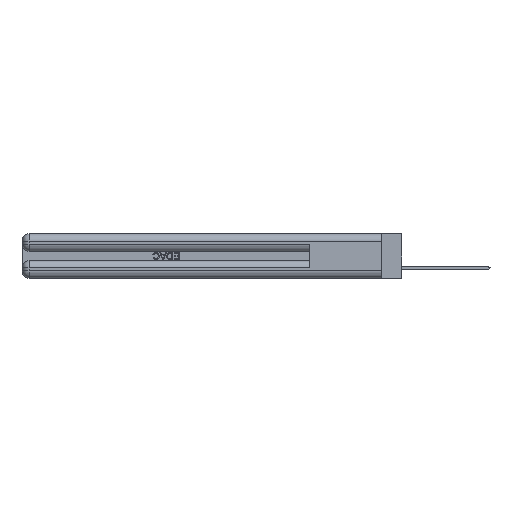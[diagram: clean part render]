
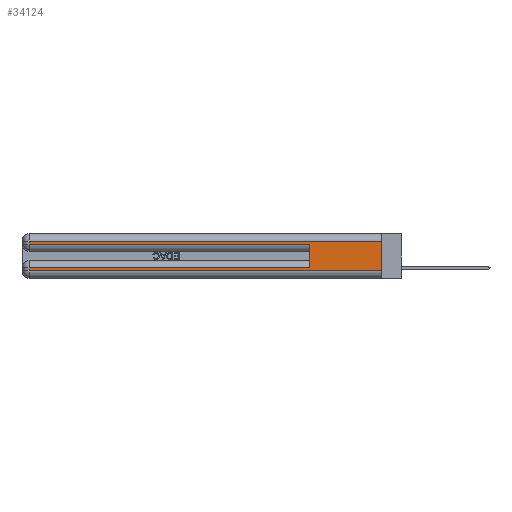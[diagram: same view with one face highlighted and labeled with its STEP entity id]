
A CAD part, left-side view. The second image highlights one B-rep face of the part: STEP entity #34124.
In plain terms, the highlighted planar face has unit normal (-1, 0, 0).
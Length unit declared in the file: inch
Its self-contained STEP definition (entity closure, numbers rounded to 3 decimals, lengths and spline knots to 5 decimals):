
#1378 = ORIENTED_EDGE ( 'NONE', *, *, #38649, .T. ) ;
#1786 = PLANE ( 'NONE',  #33733 ) ;
#1839 = CARTESIAN_POINT ( 'NONE',  ( 0., 2.94, 0.06 ) ) ;
#2216 = CARTESIAN_POINT ( 'NONE',  ( 0., 2.94, 0.085 ) ) ;
#2535 = ORIENTED_EDGE ( 'NONE', *, *, #29352, .T. ) ;
#3140 = CARTESIAN_POINT ( 'NONE',  ( 0., 0., 0.31 ) ) ;
#3660 = EDGE_CURVE ( 'NONE', #37963, #29815, #36804, .T. ) ;
#3830 = LINE ( 'NONE', #30878, #46070 ) ;
#4419 = EDGE_CURVE ( 'NONE', #34968, #53987, #10889, .T. ) ;
#8292 = VECTOR ( 'NONE', #16540, 39.37008 ) ;
#9470 = LINE ( 'NONE', #28922, #42592 ) ;
#9573 = CARTESIAN_POINT ( 'NONE',  ( 0., 0., 0.37 ) ) ;
#10889 = LINE ( 'NONE', #39249, #31305 ) ;
#11936 = ORIENTED_EDGE ( 'NONE', *, *, #4419, .T. ) ;
#14528 = LINE ( 'NONE', #39163, #37099 ) ;
#14669 = LINE ( 'NONE', #28330, #44414 ) ;
#15636 = ORIENTED_EDGE ( 'NONE', *, *, #41335, .F. ) ;
#16416 = VECTOR ( 'NONE', #32673, 39.37008 ) ;
#16540 = DIRECTION ( 'NONE',  ( 0., 0., 1. ) ) ;
#18145 = VECTOR ( 'NONE', #20030, 39.37008 ) ;
#18270 = DIRECTION ( 'NONE',  ( 0., -1., 0. ) ) ;
#20030 = DIRECTION ( 'NONE',  ( 0., 0., -1. ) ) ;
#20517 = CARTESIAN_POINT ( 'NONE',  ( 0., 0., 0.06 ) ) ;
#21413 = CARTESIAN_POINT ( 'NONE',  ( 0., 2.94, 0.31 ) ) ;
#21674 = ORIENTED_EDGE ( 'NONE', *, *, #27051, .F. ) ;
#23473 = CARTESIAN_POINT ( 'NONE',  ( 0., 0., 0.085 ) ) ;
#25510 = LINE ( 'NONE', #36879, #8292 ) ;
#26405 = VERTEX_POINT ( 'NONE', #37808 ) ;
#27051 = EDGE_CURVE ( 'NONE', #26405, #41528, #25510, .T. ) ;
#28330 = CARTESIAN_POINT ( 'NONE',  ( 0., 0., 0.31 ) ) ;
#28922 = CARTESIAN_POINT ( 'NONE',  ( 0., 2.94, 0.37 ) ) ;
#29352 = EDGE_CURVE ( 'NONE', #34262, #34968, #9470, .T. ) ;
#29815 = VERTEX_POINT ( 'NONE', #29871 ) ;
#29871 = CARTESIAN_POINT ( 'NONE',  ( 0., 2.94, 0.285 ) ) ;
#30313 = EDGE_CURVE ( 'NONE', #31188, #37963, #14669, .T. ) ;
#30878 = CARTESIAN_POINT ( 'NONE',  ( 0., 0., 0.285 ) ) ;
#31188 = VERTEX_POINT ( 'NONE', #3140 ) ;
#31305 = VECTOR ( 'NONE', #52296, 39.37008 ) ;
#32673 = DIRECTION ( 'NONE',  ( 0., 1., 0. ) ) ;
#33733 = AXIS2_PLACEMENT_3D ( 'NONE', #9573, #34882, #39119 ) ;
#34124 = ADVANCED_FACE ( 'NONE', ( #53165 ), #1786, .F. ) ;
#34262 = VERTEX_POINT ( 'NONE', #2216 ) ;
#34748 = EDGE_LOOP ( 'NONE', ( #15636, #39373, #43340, #38386, #21674, #1378, #2535, #11936 ) ) ;
#34882 = DIRECTION ( 'NONE',  ( 1., 0., 0. ) ) ;
#34968 = VERTEX_POINT ( 'NONE', #1839 ) ;
#35446 = LINE ( 'NONE', #23473, #16416 ) ;
#36804 = LINE ( 'NONE', #53652, #18145 ) ;
#36879 = CARTESIAN_POINT ( 'NONE',  ( 0., 0.6, 0.145 ) ) ;
#37099 = VECTOR ( 'NONE', #43397, 39.37008 ) ;
#37184 = DIRECTION ( 'NONE',  ( 0., 1., 0. ) ) ;
#37808 = CARTESIAN_POINT ( 'NONE',  ( 0., 0.6, 0.085 ) ) ;
#37963 = VERTEX_POINT ( 'NONE', #21413 ) ;
#38386 = ORIENTED_EDGE ( 'NONE', *, *, #49938, .T. ) ;
#38649 = EDGE_CURVE ( 'NONE', #26405, #34262, #35446, .T. ) ;
#39119 = DIRECTION ( 'NONE',  ( 0., 0., -1. ) ) ;
#39163 = CARTESIAN_POINT ( 'NONE',  ( 0., 0., 0.37 ) ) ;
#39249 = CARTESIAN_POINT ( 'NONE',  ( 0., 0., 0.06 ) ) ;
#39373 = ORIENTED_EDGE ( 'NONE', *, *, #30313, .T. ) ;
#41335 = EDGE_CURVE ( 'NONE', #31188, #53987, #14528, .T. ) ;
#41528 = VERTEX_POINT ( 'NONE', #47318 ) ;
#42592 = VECTOR ( 'NONE', #49908, 39.37008 ) ;
#43340 = ORIENTED_EDGE ( 'NONE', *, *, #3660, .T. ) ;
#43397 = DIRECTION ( 'NONE',  ( 0., 0., -1. ) ) ;
#44414 = VECTOR ( 'NONE', #37184, 39.37008 ) ;
#46070 = VECTOR ( 'NONE', #18270, 39.37008 ) ;
#47318 = CARTESIAN_POINT ( 'NONE',  ( 0., 0.6, 0.285 ) ) ;
#49908 = DIRECTION ( 'NONE',  ( 0., 0., -1. ) ) ;
#49938 = EDGE_CURVE ( 'NONE', #29815, #41528, #3830, .T. ) ;
#52296 = DIRECTION ( 'NONE',  ( 0., -1., 0. ) ) ;
#53165 = FACE_OUTER_BOUND ( 'NONE', #34748, .T. ) ;
#53652 = CARTESIAN_POINT ( 'NONE',  ( 0., 2.94, 0.37 ) ) ;
#53987 = VERTEX_POINT ( 'NONE', #20517 ) ;
